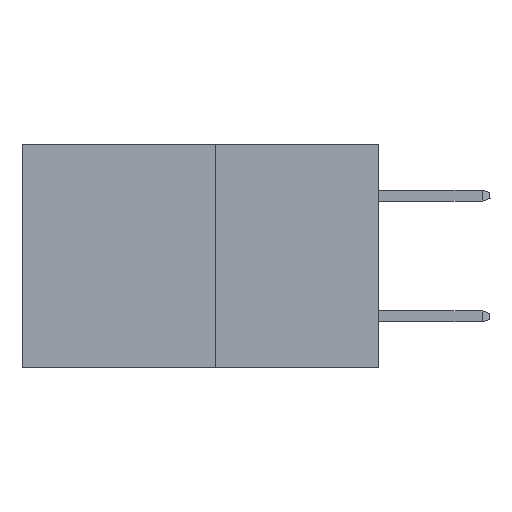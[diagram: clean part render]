
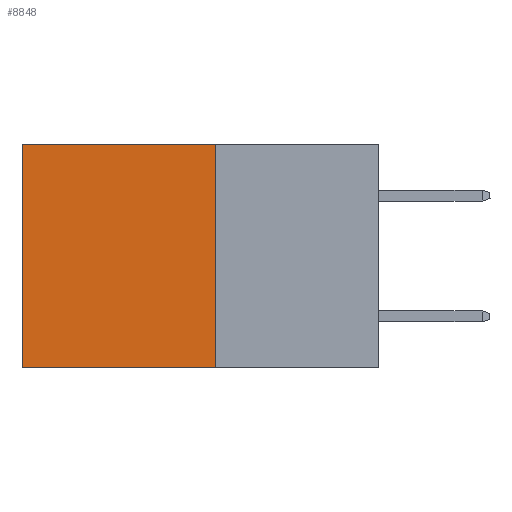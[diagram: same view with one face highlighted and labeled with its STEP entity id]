
A CAD part, left-side view. The second image highlights one B-rep face of the part: STEP entity #8848.
In plain terms, the highlighted planar face has unit normal (-1, 0, 0).
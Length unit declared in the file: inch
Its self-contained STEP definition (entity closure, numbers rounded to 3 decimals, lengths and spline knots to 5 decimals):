
#1771 = LINE ( 'NONE', #14004, #7273 ) ;
#3222 = CARTESIAN_POINT ( 'NONE',  ( 0.277, 0.27, -0.37 ) ) ;
#5239 = VERTEX_POINT ( 'NONE', #27838 ) ;
#6039 = DIRECTION ( 'NONE',  ( 0., 1., 0. ) ) ;
#6044 = PLANE ( 'NONE',  #21442 ) ;
#7273 = VECTOR ( 'NONE', #11510, 39.37008 ) ;
#7364 = ORIENTED_EDGE ( 'NONE', *, *, #26945, .F. ) ;
#8753 = CARTESIAN_POINT ( 'NONE',  ( 0.277, 0.27, -0.37 ) ) ;
#8754 = DIRECTION ( 'NONE',  ( 0., 0., -1. ) ) ;
#8848 = ADVANCED_FACE ( 'NONE', ( #23886 ), #6044, .F. ) ;
#9539 = EDGE_CURVE ( 'NONE', #31730, #22391, #1771, .T. ) ;
#10811 = ORIENTED_EDGE ( 'NONE', *, *, #32117, .T. ) ;
#11510 = DIRECTION ( 'NONE',  ( 0., 0., -1. ) ) ;
#11591 = CARTESIAN_POINT ( 'NONE',  ( 0.277, 0.27, -0.37 ) ) ;
#11641 = VECTOR ( 'NONE', #29822, 39.37008 ) ;
#13569 = EDGE_LOOP ( 'NONE', ( #17788, #30547, #7364, #10811 ) ) ;
#14004 = CARTESIAN_POINT ( 'NONE',  ( 0.277, 0.59, -0.37 ) ) ;
#14040 = CARTESIAN_POINT ( 'NONE',  ( 0.277, 0.27, 0. ) ) ;
#14318 = DIRECTION ( 'NONE',  ( 0., 1., 0. ) ) ;
#15044 = VECTOR ( 'NONE', #6039, 39.37008 ) ;
#16927 = LINE ( 'NONE', #11591, #23134 ) ;
#17323 = CARTESIAN_POINT ( 'NONE',  ( 0.277, 0.59, -0.37 ) ) ;
#17788 = ORIENTED_EDGE ( 'NONE', *, *, #9539, .T. ) ;
#19578 = CARTESIAN_POINT ( 'NONE',  ( 0.277, 0.59, 0. ) ) ;
#21442 = AXIS2_PLACEMENT_3D ( 'NONE', #22063, #24690, #8754 ) ;
#22063 = CARTESIAN_POINT ( 'NONE',  ( 0.277, 0.27, -0.37 ) ) ;
#22391 = VERTEX_POINT ( 'NONE', #17323 ) ;
#23134 = VECTOR ( 'NONE', #14318, 39.37008 ) ;
#23886 = FACE_OUTER_BOUND ( 'NONE', #13569, .T. ) ;
#24690 = DIRECTION ( 'NONE',  ( 1., 0., 0. ) ) ;
#26945 = EDGE_CURVE ( 'NONE', #5239, #26978, #27430, .T. ) ;
#26978 = VERTEX_POINT ( 'NONE', #8753 ) ;
#27430 = LINE ( 'NONE', #3222, #11641 ) ;
#27838 = CARTESIAN_POINT ( 'NONE',  ( 0.277, 0.27, 0. ) ) ;
#28251 = EDGE_CURVE ( 'NONE', #26978, #22391, #16927, .T. ) ;
#29040 = LINE ( 'NONE', #14040, #15044 ) ;
#29822 = DIRECTION ( 'NONE',  ( 0., 0., -1. ) ) ;
#30547 = ORIENTED_EDGE ( 'NONE', *, *, #28251, .F. ) ;
#31730 = VERTEX_POINT ( 'NONE', #19578 ) ;
#32117 = EDGE_CURVE ( 'NONE', #5239, #31730, #29040, .T. ) ;
